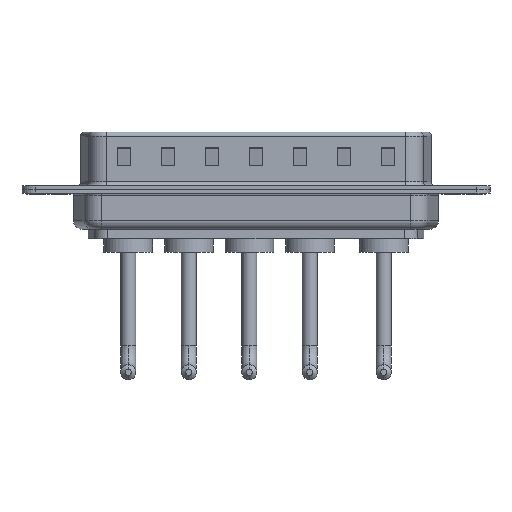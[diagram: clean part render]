
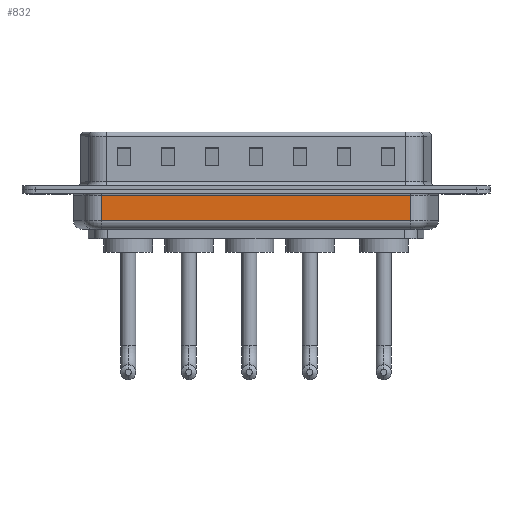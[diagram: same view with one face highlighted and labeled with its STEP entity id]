
A CAD part, front view. The second image highlights one B-rep face of the part: STEP entity #832.
In plain terms, the highlighted planar face has unit normal (0, -1, 0).
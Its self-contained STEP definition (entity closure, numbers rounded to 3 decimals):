
#59 = ORIENTED_EDGE ( 'NONE', *, *, #9117, .T. ) ;
#359 = CARTESIAN_POINT ( 'NONE',  ( 41.044, -5.35, -4.5 ) ) ;
#782 = LINE ( 'NONE', #2573, #7329 ) ;
#832 = ADVANCED_FACE ( 'NONE', ( #7144 ), #8033, .F. ) ;
#1505 = AXIS2_PLACEMENT_3D ( 'NONE', #9198, #5178, #6174 ) ;
#2573 = CARTESIAN_POINT ( 'NONE',  ( 6.006, -5.35, -4.5 ) ) ;
#3008 = VECTOR ( 'NONE', #8887, 1000. ) ;
#3149 = LINE ( 'NONE', #11784, #3714 ) ;
#3665 = EDGE_CURVE ( 'NONE', #10477, #5944, #3149, .T. ) ;
#3714 = VECTOR ( 'NONE', #7901, 1000. ) ;
#4518 = ORIENTED_EDGE ( 'NONE', *, *, #10838, .T. ) ;
#4742 = LINE ( 'NONE', #6707, #10580 ) ;
#5178 = DIRECTION ( 'NONE',  ( 0., 1., 0. ) ) ;
#5179 = LINE ( 'NONE', #359, #3008 ) ;
#5450 = CARTESIAN_POINT ( 'NONE',  ( 41.044, -5.35, -3.5 ) ) ;
#5944 = VERTEX_POINT ( 'NONE', #5450 ) ;
#6174 = DIRECTION ( 'NONE',  ( 0., 0., 1. ) ) ;
#6684 = ORIENTED_EDGE ( 'NONE', *, *, #3665, .T. ) ;
#6707 = CARTESIAN_POINT ( 'NONE',  ( 6.006, -5.35, -0.65 ) ) ;
#6843 = EDGE_LOOP ( 'NONE', ( #9443, #6684, #59, #4518 ) ) ;
#7144 = FACE_OUTER_BOUND ( 'NONE', #6843, .T. ) ;
#7329 = VECTOR ( 'NONE', #7393, 1000. ) ;
#7393 = DIRECTION ( 'NONE',  ( 0., 0., 1. ) ) ;
#7436 = CARTESIAN_POINT ( 'NONE',  ( 41.044, -5.35, -0.65 ) ) ;
#7661 = DIRECTION ( 'NONE',  ( -1., 0., 0. ) ) ;
#7901 = DIRECTION ( 'NONE',  ( 1., 0., 0. ) ) ;
#8033 = PLANE ( 'NONE',  #1505 ) ;
#8500 = CARTESIAN_POINT ( 'NONE',  ( 6.006, -5.35, -0.65 ) ) ;
#8887 = DIRECTION ( 'NONE',  ( 0., 0., 1. ) ) ;
#9034 = CARTESIAN_POINT ( 'NONE',  ( 6.006, -5.35, -3.5 ) ) ;
#9117 = EDGE_CURVE ( 'NONE', #5944, #11046, #5179, .T. ) ;
#9198 = CARTESIAN_POINT ( 'NONE',  ( 6.006, -5.35, -4.5 ) ) ;
#9443 = ORIENTED_EDGE ( 'NONE', *, *, #12402, .F. ) ;
#10268 = VERTEX_POINT ( 'NONE', #8500 ) ;
#10477 = VERTEX_POINT ( 'NONE', #9034 ) ;
#10580 = VECTOR ( 'NONE', #7661, 1000. ) ;
#10838 = EDGE_CURVE ( 'NONE', #11046, #10268, #4742, .T. ) ;
#11046 = VERTEX_POINT ( 'NONE', #7436 ) ;
#11784 = CARTESIAN_POINT ( 'NONE',  ( 6.006, -5.35, -3.5 ) ) ;
#12402 = EDGE_CURVE ( 'NONE', #10477, #10268, #782, .T. ) ;
